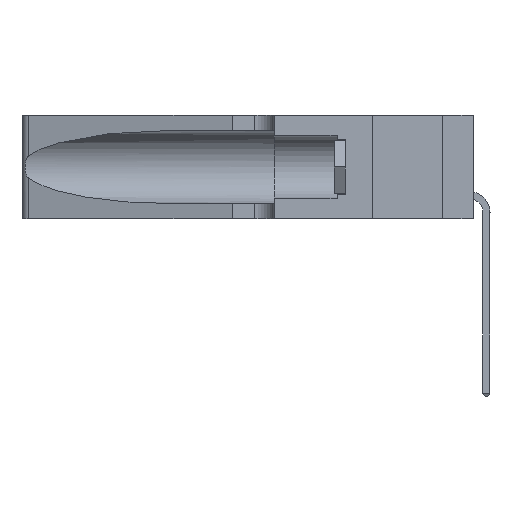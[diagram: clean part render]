
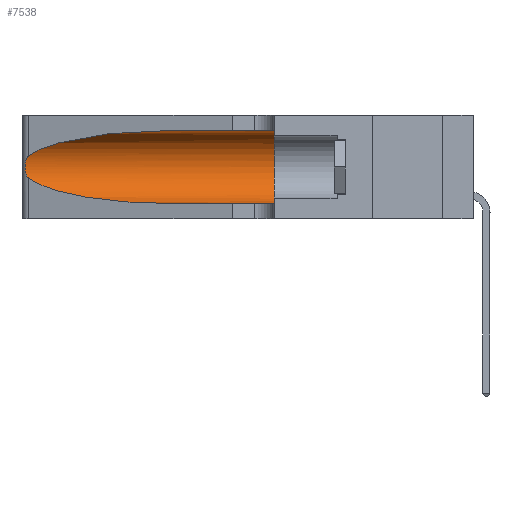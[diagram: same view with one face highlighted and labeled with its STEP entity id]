
A CAD part, left-side view. The second image highlights one B-rep face of the part: STEP entity #7538.
In plain terms, the highlighted cylindrical face has radius 3.308 mm (diameter 6.617 mm), a partial arc.
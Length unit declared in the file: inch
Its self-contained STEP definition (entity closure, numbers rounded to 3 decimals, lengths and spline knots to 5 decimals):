
#505 = DIRECTION ( 'NONE',  ( 0., -1., 0. ) ) ;
#534 = EDGE_CURVE ( 'NONE', #13941, #17066, #6852, .T. ) ;
#972 = EDGE_LOOP ( 'NONE', ( #3832, #9476, #6888, #5050, #1414, #15481 ) ) ;
#1290 = EDGE_CURVE ( 'NONE', #2645, #13620, #17104, .T. ) ;
#1414 = ORIENTED_EDGE ( 'NONE', *, *, #12922, .F. ) ;
#1526 = CARTESIAN_POINT ( 'NONE',  ( 0.25856, 1.23593, 0.16098 ) ) ;
#1601 = CARTESIAN_POINT ( 'NONE',  ( 0.26075, 1.23896, 0.178 ) ) ;
#2184 = DIRECTION ( 'NONE',  ( 0., 0., -1. ) ) ;
#2490 = CARTESIAN_POINT ( 'NONE',  ( 0.25487, 1.22718, 0.14631 ) ) ;
#2550 = CARTESIAN_POINT ( 'NONE',  ( 0.1305, 0.72297, 0.31525 ) ) ;
#2645 = VERTEX_POINT ( 'NONE', #12587 ) ;
#3061 = VECTOR ( 'NONE', #8484, 39.37008 ) ;
#3309 = CARTESIAN_POINT ( 'NONE',  ( 0.1305, 1.61858, 0.31525 ) ) ;
#3727 = DIRECTION ( 'NONE',  ( 0., 1., 0. ) ) ;
#3832 = ORIENTED_EDGE ( 'NONE', *, *, #11599, .T. ) ;
#3854 = CARTESIAN_POINT ( 'NONE',  ( 0.25487, 1.22718, 0.22369 ) ) ;
#4685 = AXIS2_PLACEMENT_3D ( 'NONE', #18111, #10818, #2184 ) ;
#5050 = ORIENTED_EDGE ( 'NONE', *, *, #16438, .T. ) ;
#5077 = CARTESIAN_POINT ( 'NONE',  ( 0.25787, 1.23484, 0.2124 ) ) ;
#5538 = EDGE_CURVE ( 'NONE', #8028, #13941, #11908, .T. ) ;
#5559 = CARTESIAN_POINT ( 'NONE',  ( 0.1305, 0.35, 0.185 ) ) ;
#6127 = CARTESIAN_POINT ( 'NONE',  ( 0.18966, 0.96281, 0.05475 ) ) ;
#6167 = CARTESIAN_POINT ( 'NONE',  ( 0.18966, 0.96281, 0.31525 ) ) ;
#6852 =( BOUNDED_CURVE ( )  B_SPLINE_CURVE ( 3, ( #11490, #13473, #6127, #18437 ),
 .UNSPECIFIED., .F., .T. ) 
 B_SPLINE_CURVE_WITH_KNOTS ( ( 4, 4 ),
 ( 3.44316, 4.71239 ),
 .UNSPECIFIED. ) 
 CURVE ( )  GEOMETRIC_REPRESENTATION_ITEM ( )  RATIONAL_B_SPLINE_CURVE ( ( 1., 0.87, 0.87, 1. ) ) 
 REPRESENTATION_ITEM ( '' )  );
#6888 = ORIENTED_EDGE ( 'NONE', *, *, #534, .T. ) ;
#7127 = FACE_OUTER_BOUND ( 'NONE', #972, .T. ) ;
#7538 = ADVANCED_FACE ( 'NONE', ( #7127 ), #12055, .F. ) ;
#8028 = VERTEX_POINT ( 'NONE', #3854 ) ;
#8484 = DIRECTION ( 'NONE',  ( 0., -1., 0. ) ) ;
#8566 = CARTESIAN_POINT ( 'NONE',  ( 0.25854, 1.2359, 0.20912 ) ) ;
#8649 = CARTESIAN_POINT ( 'NONE',  ( 0.25639, 1.23184, 0.21858 ) ) ;
#8817 = CIRCLE ( 'NONE', #12245, 0.13025 ) ;
#9476 = ORIENTED_EDGE ( 'NONE', *, *, #5538, .T. ) ;
#10320 = CARTESIAN_POINT ( 'NONE',  ( 0.26017, 1.23833, 0.17102 ) ) ;
#10818 = DIRECTION ( 'NONE',  ( 0., -1., 0. ) ) ;
#11490 = CARTESIAN_POINT ( 'NONE',  ( 0.25487, 1.22718, 0.14631 ) ) ;
#11599 = EDGE_CURVE ( 'NONE', #2645, #8028, #12314, .T. ) ;
#11908 = B_SPLINE_CURVE_WITH_KNOTS ( 'NONE', 3,
 ( #19101, #15609, #8649, #5077, #8566, #17385, #20890, #1601, #10320, #1526, #13921, #20970, #15686, #2490 ),
 .UNSPECIFIED., .F., .F.,
 ( 4, 2, 2, 2, 2, 2, 4 ),
 ( 0., 0.00027, 0.00053, 0.00107, 0.0016, 0.00187, 0.00214 ),
 .UNSPECIFIED. ) ;
#12036 = CARTESIAN_POINT ( 'NONE',  ( 0.1305, 0.72297, 0.05475 ) ) ;
#12055 = CYLINDRICAL_SURFACE ( 'NONE', #4685, 0.13025 ) ;
#12245 = AXIS2_PLACEMENT_3D ( 'NONE', #5559, #3727, #14326 ) ;
#12314 =( BOUNDED_CURVE ( )  B_SPLINE_CURVE ( 3, ( #2550, #6167, #18476, #16628 ),
 .UNSPECIFIED., .F., .F. ) 
 B_SPLINE_CURVE_WITH_KNOTS ( ( 4, 4 ),
 ( 1.5708, 2.84003 ),
 .UNSPECIFIED. ) 
 CURVE ( )  GEOMETRIC_REPRESENTATION_ITEM ( )  RATIONAL_B_SPLINE_CURVE ( ( 1., 0.87, 0.87, 1. ) ) 
 REPRESENTATION_ITEM ( '' )  );
#12587 = CARTESIAN_POINT ( 'NONE',  ( 0.1305, 0.72297, 0.31525 ) ) ;
#12674 = VERTEX_POINT ( 'NONE', #20792 ) ;
#12922 = EDGE_CURVE ( 'NONE', #13620, #12674, #8817, .T. ) ;
#13116 = LINE ( 'NONE', #19908, #19474 ) ;
#13473 = CARTESIAN_POINT ( 'NONE',  ( 0.2373, 1.15595, 0.08982 ) ) ;
#13620 = VERTEX_POINT ( 'NONE', #19987 ) ;
#13753 = CARTESIAN_POINT ( 'NONE',  ( 0.25487, 1.22718, 0.14631 ) ) ;
#13921 = CARTESIAN_POINT ( 'NONE',  ( 0.25789, 1.23486, 0.15765 ) ) ;
#13941 = VERTEX_POINT ( 'NONE', #13753 ) ;
#14326 = DIRECTION ( 'NONE',  ( 0., 0., 1. ) ) ;
#15481 = ORIENTED_EDGE ( 'NONE', *, *, #1290, .F. ) ;
#15609 = CARTESIAN_POINT ( 'NONE',  ( 0.25555, 1.22994, 0.2215 ) ) ;
#15686 = CARTESIAN_POINT ( 'NONE',  ( 0.25555, 1.22993, 0.14849 ) ) ;
#16438 = EDGE_CURVE ( 'NONE', #17066, #12674, #13116, .T. ) ;
#16628 = CARTESIAN_POINT ( 'NONE',  ( 0.25487, 1.22718, 0.22369 ) ) ;
#17066 = VERTEX_POINT ( 'NONE', #12036 ) ;
#17104 = LINE ( 'NONE', #3309, #3061 ) ;
#17385 = CARTESIAN_POINT ( 'NONE',  ( 0.26018, 1.23835, 0.19895 ) ) ;
#18111 = CARTESIAN_POINT ( 'NONE',  ( 0.1305, 1.61858, 0.185 ) ) ;
#18437 = CARTESIAN_POINT ( 'NONE',  ( 0.1305, 0.72297, 0.05475 ) ) ;
#18476 = CARTESIAN_POINT ( 'NONE',  ( 0.2373, 1.15595, 0.28018 ) ) ;
#19101 = CARTESIAN_POINT ( 'NONE',  ( 0.25487, 1.22718, 0.22369 ) ) ;
#19474 = VECTOR ( 'NONE', #505, 39.37008 ) ;
#19908 = CARTESIAN_POINT ( 'NONE',  ( 0.1305, 1.61858, 0.05475 ) ) ;
#19987 = CARTESIAN_POINT ( 'NONE',  ( 0.1305, 0.35, 0.31525 ) ) ;
#20792 = CARTESIAN_POINT ( 'NONE',  ( 0.1305, 0.35, 0.05475 ) ) ;
#20890 = CARTESIAN_POINT ( 'NONE',  ( 0.26075, 1.23896, 0.19203 ) ) ;
#20970 = CARTESIAN_POINT ( 'NONE',  ( 0.25639, 1.23186, 0.15144 ) ) ;
